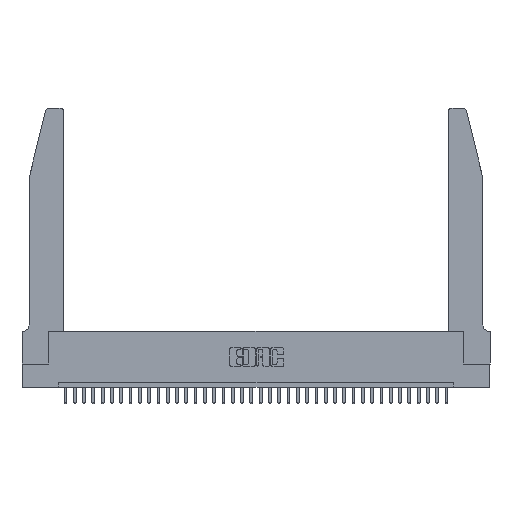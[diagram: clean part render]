
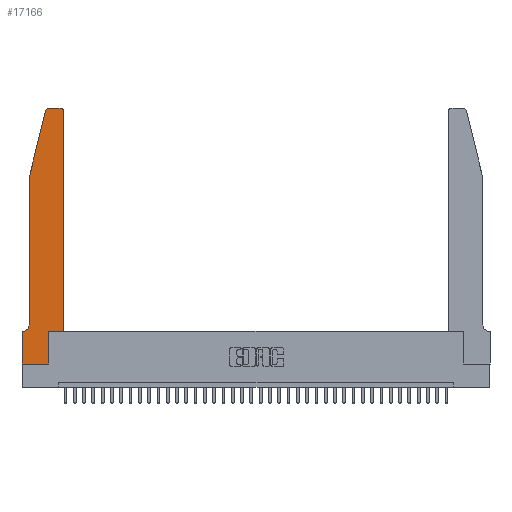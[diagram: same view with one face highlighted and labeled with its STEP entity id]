
A CAD part, top view. The second image highlights one B-rep face of the part: STEP entity #17166.
In plain terms, the highlighted planar face has unit normal (0, 0, 1).
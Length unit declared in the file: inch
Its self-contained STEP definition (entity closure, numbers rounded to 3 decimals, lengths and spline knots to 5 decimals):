
#300 = ORIENTED_EDGE ( 'NONE', *, *, #14998, .T. ) ;
#486 = VECTOR ( 'NONE', #27267, 39.37008 ) ;
#816 = VERTEX_POINT ( 'NONE', #22181 ) ;
#1170 = CARTESIAN_POINT ( 'NONE',  ( 0.4205, 2.75, 0.37 ) ) ;
#1377 = ORIENTED_EDGE ( 'NONE', *, *, #23236, .T. ) ;
#1460 = LINE ( 'NONE', #34010, #26983 ) ;
#1482 = VECTOR ( 'NONE', #28185, 39.37008 ) ;
#2300 = CARTESIAN_POINT ( 'NONE',  ( 0.4205, 2.72, 0.37 ) ) ;
#2442 = EDGE_CURVE ( 'NONE', #816, #35209, #17568, .T. ) ;
#2883 = EDGE_CURVE ( 'NONE', #30835, #31630, #7864, .T. ) ;
#3447 = DIRECTION ( 'NONE',  ( -0.239, -0.971, 0. ) ) ;
#3977 = LINE ( 'NONE', #12844, #486 ) ;
#4858 = DIRECTION ( 'NONE',  ( 0., 1., 0. ) ) ;
#4944 = DIRECTION ( 'NONE',  ( 0., 0., 1. ) ) ;
#4999 = DIRECTION ( 'NONE',  ( 0., 0., 1. ) ) ;
#6134 = VECTOR ( 'NONE', #3447, 39.37008 ) ;
#6978 = LINE ( 'NONE', #36168, #14444 ) ;
#7446 = VECTOR ( 'NONE', #33893, 39.37008 ) ;
#7593 = ORIENTED_EDGE ( 'NONE', *, *, #2442, .T. ) ;
#7864 = CIRCLE ( 'NONE', #30200, 0.03 ) ;
#7929 = DIRECTION ( 'NONE',  ( 0., 0., 1. ) ) ;
#9597 = DIRECTION ( 'NONE',  ( 1., 0., 0. ) ) ;
#9980 = EDGE_LOOP ( 'NONE', ( #16347, #20437, #23459, #7593, #33816, #1377, #34715, #13946, #17349, #27603, #25534, #300 ) ) ;
#10005 = CARTESIAN_POINT ( 'NONE',  ( 0.2865, 0., 0.37 ) ) ;
#10193 = EDGE_CURVE ( 'NONE', #26642, #30835, #3977, .T. ) ;
#10742 = CARTESIAN_POINT ( 'NONE',  ( 0.284, 2.72, 0.37 ) ) ;
#11346 = EDGE_CURVE ( 'NONE', #31630, #816, #34319, .T. ) ;
#11592 = DIRECTION ( 'NONE',  ( -1., 0., 0. ) ) ;
#12844 = CARTESIAN_POINT ( 'NONE',  ( 0.2605, 2.75, 0.37 ) ) ;
#12886 = CARTESIAN_POINT ( 'NONE',  ( 0.4505, 2.72, 0.37 ) ) ;
#13123 = CARTESIAN_POINT ( 'NONE',  ( 0.2865, 0.35, 0.37 ) ) ;
#13946 = ORIENTED_EDGE ( 'NONE', *, *, #34369, .T. ) ;
#14173 = AXIS2_PLACEMENT_3D ( 'NONE', #2300, #7929, #21995 ) ;
#14444 = VECTOR ( 'NONE', #19264, 39.37008 ) ;
#14671 = CARTESIAN_POINT ( 'NONE',  ( 0.0055, 0.42, 0.37 ) ) ;
#14998 = EDGE_CURVE ( 'NONE', #22350, #26642, #21271, .T. ) ;
#15159 = CARTESIAN_POINT ( 'NONE',  ( 0.284, 2.75, 0.37 ) ) ;
#15269 = EDGE_CURVE ( 'NONE', #35209, #22731, #16387, .T. ) ;
#15679 = CARTESIAN_POINT ( 'NONE',  ( 0.4505, 0.35, 0.37 ) ) ;
#15773 = CARTESIAN_POINT ( 'NONE',  ( 0., 0.35, 0.37 ) ) ;
#15984 = CARTESIAN_POINT ( 'NONE',  ( 0.25487, 2.72718, 0.37 ) ) ;
#16173 = VERTEX_POINT ( 'NONE', #32344 ) ;
#16347 = ORIENTED_EDGE ( 'NONE', *, *, #10193, .T. ) ;
#16387 = CIRCLE ( 'NONE', #28098, 0.07 ) ;
#17166 = ADVANCED_FACE ( 'NONE', ( #18462 ), #24413, .T. ) ;
#17349 = ORIENTED_EDGE ( 'NONE', *, *, #23844, .T. ) ;
#17399 = DIRECTION ( 'NONE',  ( 0., 0., -1. ) ) ;
#17549 = CARTESIAN_POINT ( 'NONE',  ( 0.0055, 0.35, 0.37 ) ) ;
#17568 = LINE ( 'NONE', #28709, #7446 ) ;
#17597 = CARTESIAN_POINT ( 'NONE',  ( 0.0755, 2., 0.37 ) ) ;
#18462 = FACE_OUTER_BOUND ( 'NONE', #9980, .T. ) ;
#18838 = DIRECTION ( 'NONE',  ( 1., 0., 0. ) ) ;
#19180 = DIRECTION ( 'NONE',  ( 0., -1., 0. ) ) ;
#19264 = DIRECTION ( 'NONE',  ( 1., 0., 0. ) ) ;
#20297 = VECTOR ( 'NONE', #4858, 39.37008 ) ;
#20437 = ORIENTED_EDGE ( 'NONE', *, *, #2883, .T. ) ;
#20714 = DIRECTION ( 'NONE',  ( -1., 0., 0. ) ) ;
#21271 = CIRCLE ( 'NONE', #14173, 0.03 ) ;
#21312 = CARTESIAN_POINT ( 'NONE',  ( 0., 0.35, 0.37 ) ) ;
#21819 = VERTEX_POINT ( 'NONE', #15679 ) ;
#21915 = CARTESIAN_POINT ( 'NONE',  ( 0., 0., 0.37 ) ) ;
#21995 = DIRECTION ( 'NONE',  ( 1., 0., 0. ) ) ;
#22106 = DIRECTION ( 'NONE',  ( 1., 0., 0. ) ) ;
#22181 = CARTESIAN_POINT ( 'NONE',  ( 0.0755, 2., 0.37 ) ) ;
#22350 = VERTEX_POINT ( 'NONE', #12886 ) ;
#22731 = VERTEX_POINT ( 'NONE', #17549 ) ;
#23236 = EDGE_CURVE ( 'NONE', #22731, #33365, #1460, .T. ) ;
#23452 = VECTOR ( 'NONE', #19180, 39.37008 ) ;
#23459 = ORIENTED_EDGE ( 'NONE', *, *, #11346, .T. ) ;
#23844 = EDGE_CURVE ( 'NONE', #32301, #29268, #27779, .T. ) ;
#24413 = PLANE ( 'NONE',  #31445 ) ;
#24865 = LINE ( 'NONE', #35001, #27934 ) ;
#25277 = EDGE_CURVE ( 'NONE', #29268, #21819, #6978, .T. ) ;
#25534 = ORIENTED_EDGE ( 'NONE', *, *, #31107, .T. ) ;
#26109 = LINE ( 'NONE', #30174, #1482 ) ;
#26642 = VERTEX_POINT ( 'NONE', #1170 ) ;
#26821 = CARTESIAN_POINT ( 'NONE',  ( 0.0755, 0.42, 0.37 ) ) ;
#26983 = VECTOR ( 'NONE', #11592, 39.37008 ) ;
#27267 = DIRECTION ( 'NONE',  ( -1., 0., 0. ) ) ;
#27603 = ORIENTED_EDGE ( 'NONE', *, *, #25277, .T. ) ;
#27779 = LINE ( 'NONE', #33020, #20297 ) ;
#27934 = VECTOR ( 'NONE', #9597, 39.37008 ) ;
#28098 = AXIS2_PLACEMENT_3D ( 'NONE', #14671, #17399, #20714 ) ;
#28185 = DIRECTION ( 'NONE',  ( 0., 1., 0. ) ) ;
#28709 = CARTESIAN_POINT ( 'NONE',  ( 0.0755, 2., 0.37 ) ) ;
#29268 = VERTEX_POINT ( 'NONE', #13123 ) ;
#30174 = CARTESIAN_POINT ( 'NONE',  ( 0.4505, 0.35, 0.37 ) ) ;
#30200 = AXIS2_PLACEMENT_3D ( 'NONE', #10742, #4999, #22106 ) ;
#30835 = VERTEX_POINT ( 'NONE', #15159 ) ;
#31107 = EDGE_CURVE ( 'NONE', #21819, #22350, #26109, .T. ) ;
#31445 = AXIS2_PLACEMENT_3D ( 'NONE', #15773, #4944, #18838 ) ;
#31630 = VERTEX_POINT ( 'NONE', #15984 ) ;
#31761 = EDGE_CURVE ( 'NONE', #33365, #16173, #34408, .T. ) ;
#32301 = VERTEX_POINT ( 'NONE', #10005 ) ;
#32344 = CARTESIAN_POINT ( 'NONE',  ( 0., 0., 0.37 ) ) ;
#33020 = CARTESIAN_POINT ( 'NONE',  ( 0.2865, 0.35, 0.37 ) ) ;
#33365 = VERTEX_POINT ( 'NONE', #21312 ) ;
#33816 = ORIENTED_EDGE ( 'NONE', *, *, #15269, .T. ) ;
#33893 = DIRECTION ( 'NONE',  ( 0., -1., 0. ) ) ;
#34010 = CARTESIAN_POINT ( 'NONE',  ( 0.0755, 0.35, 0.37 ) ) ;
#34319 = LINE ( 'NONE', #17597, #6134 ) ;
#34369 = EDGE_CURVE ( 'NONE', #16173, #32301, #24865, .T. ) ;
#34408 = LINE ( 'NONE', #21915, #23452 ) ;
#34715 = ORIENTED_EDGE ( 'NONE', *, *, #31761, .T. ) ;
#35001 = CARTESIAN_POINT ( 'NONE',  ( 0., 0., 0.37 ) ) ;
#35209 = VERTEX_POINT ( 'NONE', #26821 ) ;
#36168 = CARTESIAN_POINT ( 'NONE',  ( 0.4505, 0.35, 0.37 ) ) ;
